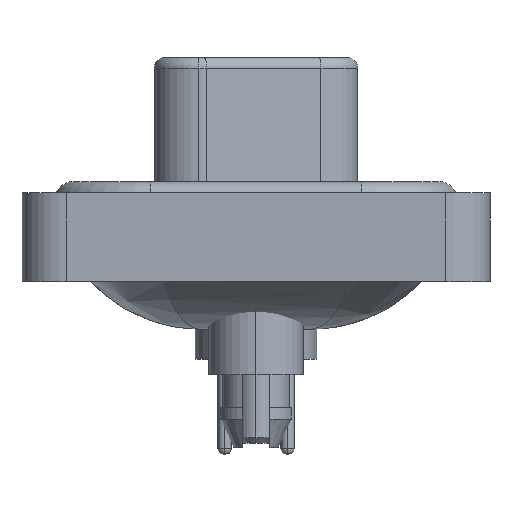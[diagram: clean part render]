
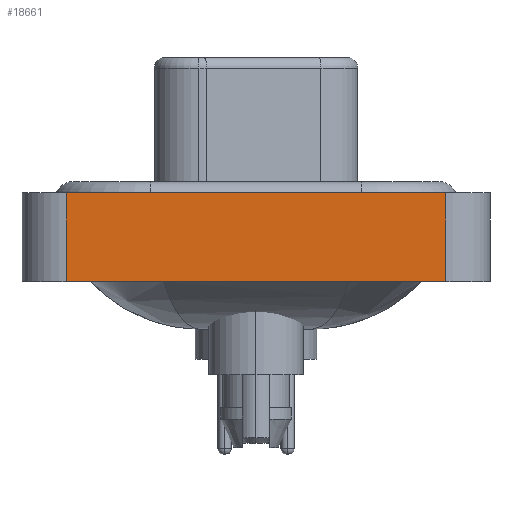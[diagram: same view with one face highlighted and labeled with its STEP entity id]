
A CAD part, left-side view. The second image highlights one B-rep face of the part: STEP entity #18661.
In plain terms, the highlighted planar face has unit normal (-1, 0, 0).
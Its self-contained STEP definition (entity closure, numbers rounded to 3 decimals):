
#834 = VECTOR ( 'NONE', #1497, 1000. ) ;
#948 = CARTESIAN_POINT ( 'NONE',  ( -7.3, -8.55, -3.6 ) ) ;
#959 = EDGE_CURVE ( 'NONE', #15236, #16472, #6421, .T. ) ;
#1379 = CARTESIAN_POINT ( 'NONE',  ( -7.3, 8.55, -3.6 ) ) ;
#1497 = DIRECTION ( 'NONE',  ( 0., -1., 0. ) ) ;
#2138 = FACE_OUTER_BOUND ( 'NONE', #12597, .T. ) ;
#2224 = CARTESIAN_POINT ( 'NONE',  ( -7.3, -8.55, -3.6 ) ) ;
#2587 = CARTESIAN_POINT ( 'NONE',  ( -7.3, -8.55, -3.6 ) ) ;
#4913 = DIRECTION ( 'NONE',  ( 0., -1., 0. ) ) ;
#5122 = EDGE_CURVE ( 'NONE', #12310, #16472, #17951, .T. ) ;
#5715 = DIRECTION ( 'NONE',  ( 0., 0., 1. ) ) ;
#6176 = VECTOR ( 'NONE', #4913, 1000. ) ;
#6421 = LINE ( 'NONE', #18848, #6176 ) ;
#6605 = ORIENTED_EDGE ( 'NONE', *, *, #959, .F. ) ;
#7040 = LINE ( 'NONE', #8972, #11453 ) ;
#8635 = CARTESIAN_POINT ( 'NONE',  ( -7.3, -8.55, 0.4 ) ) ;
#8972 = CARTESIAN_POINT ( 'NONE',  ( -7.3, 8.55, -3.6 ) ) ;
#9807 = DIRECTION ( 'NONE',  ( 0., 0., 1. ) ) ;
#9950 = PLANE ( 'NONE',  #15308 ) ;
#11453 = VECTOR ( 'NONE', #5715, 1000. ) ;
#12196 = ORIENTED_EDGE ( 'NONE', *, *, #5122, .T. ) ;
#12310 = VERTEX_POINT ( 'NONE', #2587 ) ;
#12538 = EDGE_CURVE ( 'NONE', #17993, #12310, #15417, .T. ) ;
#12597 = EDGE_LOOP ( 'NONE', ( #12196, #6605, #14726, #17350 ) ) ;
#14038 = CARTESIAN_POINT ( 'NONE',  ( -7.3, 8.55, 0.4 ) ) ;
#14726 = ORIENTED_EDGE ( 'NONE', *, *, #18355, .F. ) ;
#15236 = VERTEX_POINT ( 'NONE', #14038 ) ;
#15308 = AXIS2_PLACEMENT_3D ( 'NONE', #2224, #16165, #17892 ) ;
#15417 = LINE ( 'NONE', #16647, #834 ) ;
#16165 = DIRECTION ( 'NONE',  ( -1., 0., 0. ) ) ;
#16472 = VERTEX_POINT ( 'NONE', #8635 ) ;
#16647 = CARTESIAN_POINT ( 'NONE',  ( -7.3, -8.55, -3.6 ) ) ;
#17350 = ORIENTED_EDGE ( 'NONE', *, *, #12538, .T. ) ;
#17584 = VECTOR ( 'NONE', #9807, 1000. ) ;
#17892 = DIRECTION ( 'NONE',  ( 0., 0., 1. ) ) ;
#17951 = LINE ( 'NONE', #948, #17584 ) ;
#17993 = VERTEX_POINT ( 'NONE', #1379 ) ;
#18355 = EDGE_CURVE ( 'NONE', #17993, #15236, #7040, .T. ) ;
#18661 = ADVANCED_FACE ( 'NONE', ( #2138 ), #9950, .T. ) ;
#18848 = CARTESIAN_POINT ( 'NONE',  ( -7.3, -8.55, 0.4 ) ) ;
